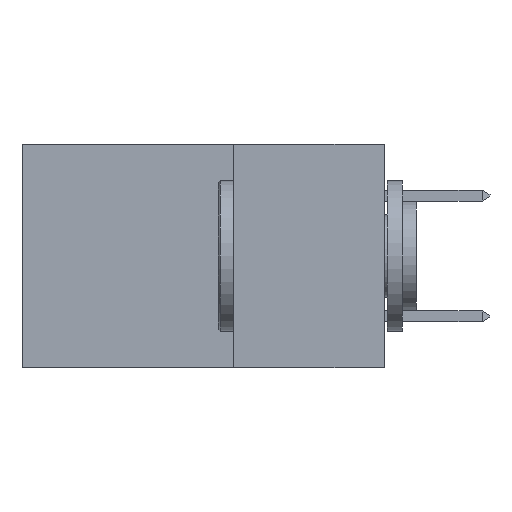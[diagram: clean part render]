
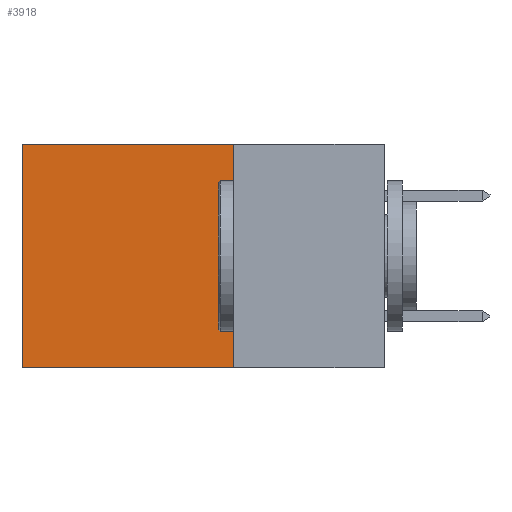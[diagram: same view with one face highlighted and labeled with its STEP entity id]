
A CAD part, left-side view. The second image highlights one B-rep face of the part: STEP entity #3918.
In plain terms, the highlighted planar face has unit normal (-1, 0, 0).
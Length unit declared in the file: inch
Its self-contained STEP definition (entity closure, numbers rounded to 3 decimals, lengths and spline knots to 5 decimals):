
#459 = CARTESIAN_POINT ( 'NONE',  ( 0.2875, 0.25, 0. ) ) ;
#646 = DIRECTION ( 'NONE',  ( 1., 0., 0. ) ) ;
#651 = DIRECTION ( 'NONE',  ( 0., 0., -1. ) ) ;
#1119 = CARTESIAN_POINT ( 'NONE',  ( 0.2875, 0.25, -0.37 ) ) ;
#1167 = VERTEX_POINT ( 'NONE', #2563 ) ;
#1852 = EDGE_CURVE ( 'NONE', #11596, #5664, #6257, .T. ) ;
#1913 = CARTESIAN_POINT ( 'NONE',  ( 0.2875, 0.25, -0.37 ) ) ;
#2248 = FACE_OUTER_BOUND ( 'NONE', #2386, .T. ) ;
#2386 = EDGE_LOOP ( 'NONE', ( #5644, #7200, #13074, #9795 ) ) ;
#2563 = CARTESIAN_POINT ( 'NONE',  ( 0.2875, 0.6, 0. ) ) ;
#2739 = LINE ( 'NONE', #1913, #13936 ) ;
#2910 = PLANE ( 'NONE',  #8997 ) ;
#3789 = DIRECTION ( 'NONE',  ( 0., 0., -1. ) ) ;
#3918 = ADVANCED_FACE ( 'NONE', ( #2248 ), #2910, .F. ) ;
#4409 = LINE ( 'NONE', #10253, #7260 ) ;
#5453 = EDGE_CURVE ( 'NONE', #5664, #7650, #2739, .T. ) ;
#5644 = ORIENTED_EDGE ( 'NONE', *, *, #8050, .T. ) ;
#5664 = VERTEX_POINT ( 'NONE', #1119 ) ;
#5829 = LINE ( 'NONE', #10384, #8677 ) ;
#6257 = LINE ( 'NONE', #11664, #9450 ) ;
#7200 = ORIENTED_EDGE ( 'NONE', *, *, #5453, .F. ) ;
#7260 = VECTOR ( 'NONE', #3789, 39.37008 ) ;
#7650 = VERTEX_POINT ( 'NONE', #10633 ) ;
#8050 = EDGE_CURVE ( 'NONE', #1167, #7650, #4409, .T. ) ;
#8677 = VECTOR ( 'NONE', #11468, 39.37008 ) ;
#8811 = EDGE_CURVE ( 'NONE', #11596, #1167, #5829, .T. ) ;
#8997 = AXIS2_PLACEMENT_3D ( 'NONE', #459, #646, #651 ) ;
#9450 = VECTOR ( 'NONE', #11578, 39.37008 ) ;
#9795 = ORIENTED_EDGE ( 'NONE', *, *, #8811, .T. ) ;
#10253 = CARTESIAN_POINT ( 'NONE',  ( 0.2875, 0.6, 0. ) ) ;
#10384 = CARTESIAN_POINT ( 'NONE',  ( 0.2875, 0.25, 0. ) ) ;
#10627 = DIRECTION ( 'NONE',  ( 0., 1., 0. ) ) ;
#10633 = CARTESIAN_POINT ( 'NONE',  ( 0.2875, 0.6, -0.37 ) ) ;
#10823 = CARTESIAN_POINT ( 'NONE',  ( 0.2875, 0.25, 0. ) ) ;
#11468 = DIRECTION ( 'NONE',  ( 0., 1., 0. ) ) ;
#11578 = DIRECTION ( 'NONE',  ( 0., 0., -1. ) ) ;
#11596 = VERTEX_POINT ( 'NONE', #10823 ) ;
#11664 = CARTESIAN_POINT ( 'NONE',  ( 0.2875, 0.25, 0. ) ) ;
#13074 = ORIENTED_EDGE ( 'NONE', *, *, #1852, .F. ) ;
#13936 = VECTOR ( 'NONE', #10627, 39.37008 ) ;
